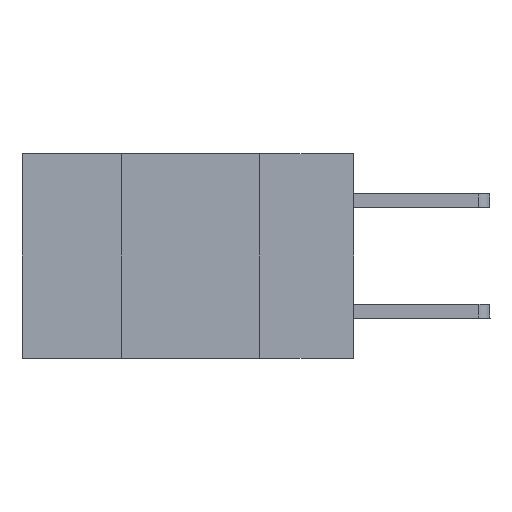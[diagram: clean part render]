
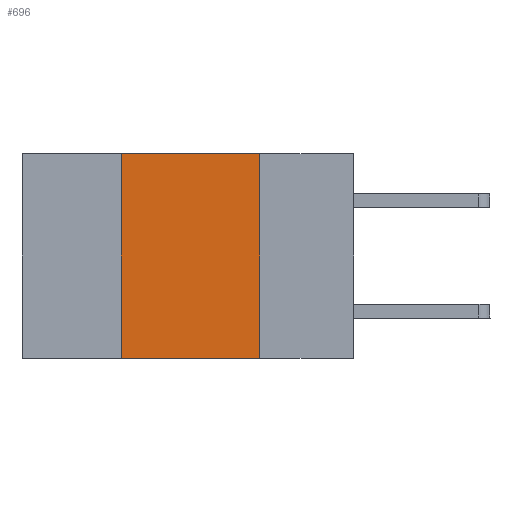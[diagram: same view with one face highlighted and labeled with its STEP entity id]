
A CAD part, left-side view. The second image highlights one B-rep face of the part: STEP entity #696.
In plain terms, the highlighted planar face has unit normal (-1, 0, 0).
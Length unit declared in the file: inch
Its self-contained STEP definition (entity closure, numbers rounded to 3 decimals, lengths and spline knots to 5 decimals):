
#134 = VECTOR ( 'NONE', #12093, 39.37008 ) ;
#441 = LINE ( 'NONE', #3466, #447 ) ;
#446 = VERTEX_POINT ( 'NONE', #5489 ) ;
#447 = VECTOR ( 'NONE', #2470, 39.37008 ) ;
#611 = AXIS2_PLACEMENT_3D ( 'NONE', #2532, #5606, #9315 ) ;
#696 = ADVANCED_FACE ( 'NONE', ( #7355 ), #11436, .F. ) ;
#834 = DIRECTION ( 'NONE',  ( 0., -1., 0. ) ) ;
#2470 = DIRECTION ( 'NONE',  ( 0., 0., 1. ) ) ;
#2532 = CARTESIAN_POINT ( 'NONE',  ( 0., 0.6, 0. ) ) ;
#3195 = EDGE_CURVE ( 'NONE', #4855, #446, #6987, .T. ) ;
#3409 = VECTOR ( 'NONE', #8033, 39.37008 ) ;
#3466 = CARTESIAN_POINT ( 'NONE',  ( 0., 0.42, 0. ) ) ;
#3808 = CARTESIAN_POINT ( 'NONE',  ( 0., 0.6, -0.37 ) ) ;
#4068 = LINE ( 'NONE', #8806, #3409 ) ;
#4423 = VERTEX_POINT ( 'NONE', #5469 ) ;
#4855 = VERTEX_POINT ( 'NONE', #10269 ) ;
#5142 = LINE ( 'NONE', #10190, #134 ) ;
#5259 = EDGE_CURVE ( 'NONE', #4855, #4423, #441, .T. ) ;
#5388 = ORIENTED_EDGE ( 'NONE', *, *, #3195, .T. ) ;
#5444 = EDGE_LOOP ( 'NONE', ( #10714, #8553, #11822, #5388 ) ) ;
#5469 = CARTESIAN_POINT ( 'NONE',  ( 0., 0.42, 0. ) ) ;
#5489 = CARTESIAN_POINT ( 'NONE',  ( 0., 0.17, -0.37 ) ) ;
#5606 = DIRECTION ( 'NONE',  ( 1., 0., 0. ) ) ;
#6155 = EDGE_CURVE ( 'NONE', #4423, #9723, #4068, .T. ) ;
#6987 = LINE ( 'NONE', #3808, #8320 ) ;
#7355 = FACE_OUTER_BOUND ( 'NONE', #5444, .T. ) ;
#8033 = DIRECTION ( 'NONE',  ( 0., -1., 0. ) ) ;
#8320 = VECTOR ( 'NONE', #834, 39.37008 ) ;
#8553 = ORIENTED_EDGE ( 'NONE', *, *, #6155, .F. ) ;
#8806 = CARTESIAN_POINT ( 'NONE',  ( 0., 0.6, 0. ) ) ;
#9315 = DIRECTION ( 'NONE',  ( 0., 0., -1. ) ) ;
#9703 = CARTESIAN_POINT ( 'NONE',  ( 0., 0.17, 0. ) ) ;
#9723 = VERTEX_POINT ( 'NONE', #9703 ) ;
#10190 = CARTESIAN_POINT ( 'NONE',  ( 0., 0.17, 0. ) ) ;
#10269 = CARTESIAN_POINT ( 'NONE',  ( 0., 0.42, -0.37 ) ) ;
#10714 = ORIENTED_EDGE ( 'NONE', *, *, #11670, .F. ) ;
#11436 = PLANE ( 'NONE',  #611 ) ;
#11670 = EDGE_CURVE ( 'NONE', #9723, #446, #5142, .T. ) ;
#11822 = ORIENTED_EDGE ( 'NONE', *, *, #5259, .F. ) ;
#12093 = DIRECTION ( 'NONE',  ( 0., 0., -1. ) ) ;
